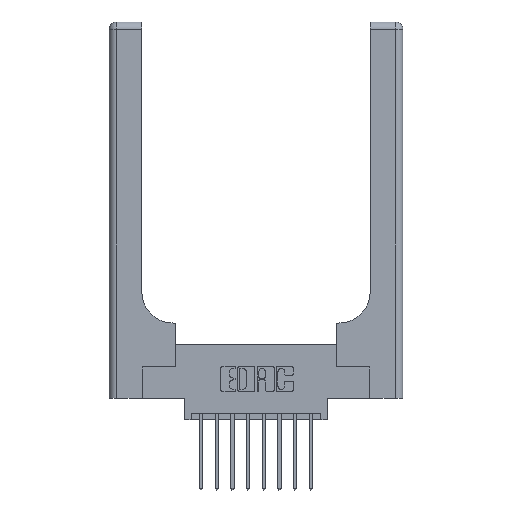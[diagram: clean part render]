
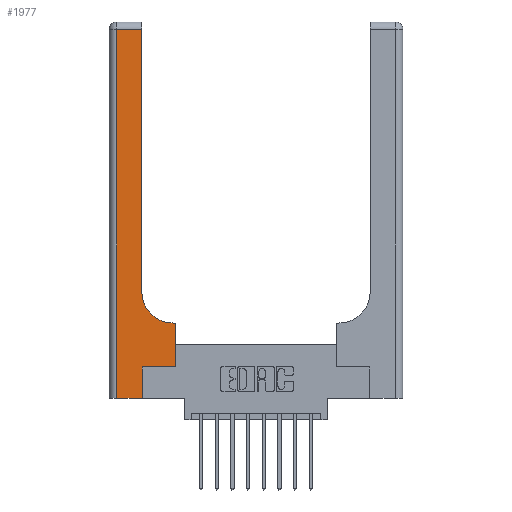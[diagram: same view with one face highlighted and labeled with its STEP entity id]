
A CAD part, top view. The second image highlights one B-rep face of the part: STEP entity #1977.
In plain terms, the highlighted planar face has unit normal (0, 0, 1).
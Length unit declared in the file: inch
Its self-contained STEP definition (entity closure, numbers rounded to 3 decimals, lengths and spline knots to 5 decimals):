
#191 = CARTESIAN_POINT ( 'NONE',  ( 0.26, 2.94, 0.37 ) ) ;
#293 = CARTESIAN_POINT ( 'NONE',  ( 0.06, 3., 0.37 ) ) ;
#465 = CARTESIAN_POINT ( 'NONE',  ( 0.528, 0.25, 0.37 ) ) ;
#482 = EDGE_LOOP ( 'NONE', ( #2975, #8938, #5599, #13182, #4039, #3257, #10351, #13676, #6420 ) ) ;
#592 = LINE ( 'NONE', #8877, #10050 ) ;
#1095 = VECTOR ( 'NONE', #3787, 39.37008 ) ;
#1175 = LINE ( 'NONE', #10906, #13672 ) ;
#1659 = CARTESIAN_POINT ( 'NONE',  ( 0.26, 3., 0.37 ) ) ;
#1977 = ADVANCED_FACE ( 'NONE', ( #3500 ), #9310, .F. ) ;
#2284 = DIRECTION ( 'NONE',  ( 1., 0., 0. ) ) ;
#2533 = CARTESIAN_POINT ( 'NONE',  ( 0.26, 0.85, 0.37 ) ) ;
#2755 = VERTEX_POINT ( 'NONE', #7864 ) ;
#2852 = EDGE_CURVE ( 'NONE', #12049, #10104, #14823, .T. ) ;
#2975 = ORIENTED_EDGE ( 'NONE', *, *, #11764, .T. ) ;
#3008 = AXIS2_PLACEMENT_3D ( 'NONE', #3584, #13086, #14101 ) ;
#3134 = CARTESIAN_POINT ( 'NONE',  ( 0.06, 0., 0.37 ) ) ;
#3198 = EDGE_CURVE ( 'NONE', #7472, #2755, #3215, .T. ) ;
#3215 = LINE ( 'NONE', #11609, #5413 ) ;
#3257 = ORIENTED_EDGE ( 'NONE', *, *, #13134, .T. ) ;
#3361 = CARTESIAN_POINT ( 'NONE',  ( 0.528, 0.25, 0.37 ) ) ;
#3500 = FACE_OUTER_BOUND ( 'NONE', #482, .T. ) ;
#3584 = CARTESIAN_POINT ( 'NONE',  ( 0., 3., 0.37 ) ) ;
#3708 = VECTOR ( 'NONE', #9750, 39.37008 ) ;
#3787 = DIRECTION ( 'NONE',  ( 0., 1., 0. ) ) ;
#4039 = ORIENTED_EDGE ( 'NONE', *, *, #12326, .T. ) ;
#4138 = EDGE_CURVE ( 'NONE', #10538, #12049, #7064, .T. ) ;
#4378 = DIRECTION ( 'NONE',  ( 0., 1., 0. ) ) ;
#4481 = EDGE_CURVE ( 'NONE', #12759, #7472, #11078, .T. ) ;
#4691 = CARTESIAN_POINT ( 'NONE',  ( 0.265, 0., 0.37 ) ) ;
#4718 = DIRECTION ( 'NONE',  ( 0., 0., -1. ) ) ;
#4881 = VERTEX_POINT ( 'NONE', #191 ) ;
#5413 = VECTOR ( 'NONE', #8084, 39.37008 ) ;
#5550 = LINE ( 'NONE', #3361, #15306 ) ;
#5599 = ORIENTED_EDGE ( 'NONE', *, *, #4481, .T. ) ;
#5937 = DIRECTION ( 'NONE',  ( 0., 1., 0. ) ) ;
#6123 = CARTESIAN_POINT ( 'NONE',  ( 0.26, 0.6, 0.37 ) ) ;
#6420 = ORIENTED_EDGE ( 'NONE', *, *, #2852, .T. ) ;
#6476 = VERTEX_POINT ( 'NONE', #465 ) ;
#7010 = AXIS2_PLACEMENT_3D ( 'NONE', #13333, #4718, #9524 ) ;
#7064 = LINE ( 'NONE', #6123, #3708 ) ;
#7472 = VERTEX_POINT ( 'NONE', #3134 ) ;
#7544 = LINE ( 'NONE', #1659, #1095 ) ;
#7637 = VECTOR ( 'NONE', #15160, 39.37008 ) ;
#7864 = CARTESIAN_POINT ( 'NONE',  ( 0.265, 0., 0.37 ) ) ;
#8084 = DIRECTION ( 'NONE',  ( 1., 0., 0. ) ) ;
#8311 = LINE ( 'NONE', #4691, #10876 ) ;
#8455 = EDGE_CURVE ( 'NONE', #4881, #12759, #592, .T. ) ;
#8877 = CARTESIAN_POINT ( 'NONE',  ( 0., 2.94, 0.37 ) ) ;
#8938 = ORIENTED_EDGE ( 'NONE', *, *, #8455, .T. ) ;
#8948 = DIRECTION ( 'NONE',  ( -1., 0., 0. ) ) ;
#9310 = PLANE ( 'NONE',  #3008 ) ;
#9524 = DIRECTION ( 'NONE',  ( 1., 0., 0. ) ) ;
#9750 = DIRECTION ( 'NONE',  ( -1., 0., 0. ) ) ;
#10050 = VECTOR ( 'NONE', #8948, 39.37008 ) ;
#10104 = VERTEX_POINT ( 'NONE', #2533 ) ;
#10351 = ORIENTED_EDGE ( 'NONE', *, *, #14417, .T. ) ;
#10538 = VERTEX_POINT ( 'NONE', #12501 ) ;
#10749 = CARTESIAN_POINT ( 'NONE',  ( 0.51, 0.6, 0.37 ) ) ;
#10876 = VECTOR ( 'NONE', #5937, 39.37008 ) ;
#10906 = CARTESIAN_POINT ( 'NONE',  ( 0.265, 0.25, 0.37 ) ) ;
#10926 = CARTESIAN_POINT ( 'NONE',  ( 0.06, 2.94, 0.37 ) ) ;
#11078 = LINE ( 'NONE', #293, #7637 ) ;
#11609 = CARTESIAN_POINT ( 'NONE',  ( 0., 0., 0.37 ) ) ;
#11764 = EDGE_CURVE ( 'NONE', #10104, #4881, #7544, .T. ) ;
#12049 = VERTEX_POINT ( 'NONE', #10749 ) ;
#12326 = EDGE_CURVE ( 'NONE', #2755, #14817, #8311, .T. ) ;
#12501 = CARTESIAN_POINT ( 'NONE',  ( 0.528, 0.6, 0.37 ) ) ;
#12759 = VERTEX_POINT ( 'NONE', #10926 ) ;
#13086 = DIRECTION ( 'NONE',  ( 0., 0., -1. ) ) ;
#13134 = EDGE_CURVE ( 'NONE', #14817, #6476, #1175, .T. ) ;
#13182 = ORIENTED_EDGE ( 'NONE', *, *, #3198, .T. ) ;
#13333 = CARTESIAN_POINT ( 'NONE',  ( 0.51, 0.85, 0.37 ) ) ;
#13672 = VECTOR ( 'NONE', #2284, 39.37008 ) ;
#13676 = ORIENTED_EDGE ( 'NONE', *, *, #4138, .T. ) ;
#14101 = DIRECTION ( 'NONE',  ( -1., 0., 0. ) ) ;
#14417 = EDGE_CURVE ( 'NONE', #6476, #10538, #5550, .T. ) ;
#14546 = CARTESIAN_POINT ( 'NONE',  ( 0.265, 0.25, 0.37 ) ) ;
#14817 = VERTEX_POINT ( 'NONE', #14546 ) ;
#14823 = CIRCLE ( 'NONE', #7010, 0.25 ) ;
#15160 = DIRECTION ( 'NONE',  ( 0., -1., 0. ) ) ;
#15306 = VECTOR ( 'NONE', #4378, 39.37008 ) ;
